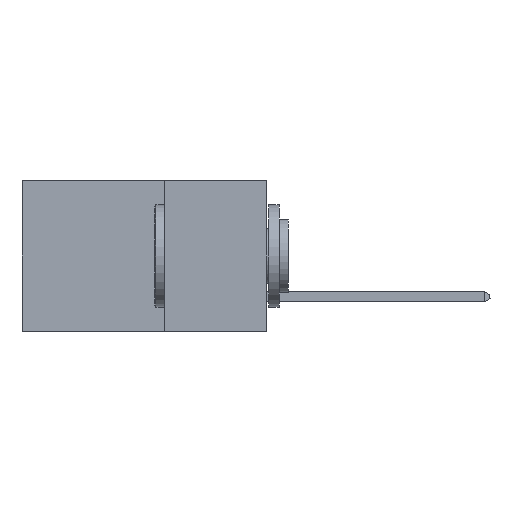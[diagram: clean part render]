
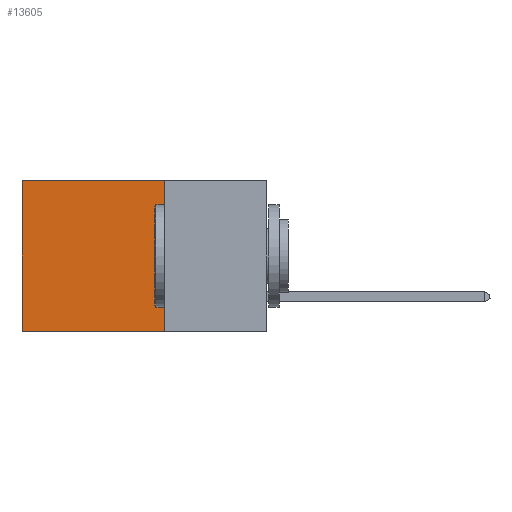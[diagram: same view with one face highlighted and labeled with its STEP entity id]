
A CAD part, left-side view. The second image highlights one B-rep face of the part: STEP entity #13605.
In plain terms, the highlighted planar face has unit normal (-1, 0, 0).
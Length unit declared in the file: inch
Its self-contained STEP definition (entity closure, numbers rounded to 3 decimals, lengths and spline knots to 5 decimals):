
#523 = FACE_OUTER_BOUND ( 'NONE', #15005, .T. ) ;
#1221 = DIRECTION ( 'NONE',  ( 1., 0., 0. ) ) ;
#2927 = LINE ( 'NONE', #26624, #24232 ) ;
#3961 = DIRECTION ( 'NONE',  ( 0., 1., 0. ) ) ;
#4845 = EDGE_CURVE ( 'NONE', #5559, #17962, #18027, .T. ) ;
#5559 = VERTEX_POINT ( 'NONE', #18708 ) ;
#5758 = AXIS2_PLACEMENT_3D ( 'NONE', #23909, #1221, #15977 ) ;
#5864 = CARTESIAN_POINT ( 'NONE',  ( 0.2875, 0.6, 0. ) ) ;
#5927 = ORIENTED_EDGE ( 'NONE', *, *, #7943, .F. ) ;
#7510 = VERTEX_POINT ( 'NONE', #18894 ) ;
#7943 = EDGE_CURVE ( 'NONE', #7510, #5559, #17322, .T. ) ;
#12088 = DIRECTION ( 'NONE',  ( 0., 0., -1. ) ) ;
#12649 = VECTOR ( 'NONE', #19004, 39.37008 ) ;
#13605 = ADVANCED_FACE ( 'NONE', ( #523 ), #15888, .F. ) ;
#15005 = EDGE_LOOP ( 'NONE', ( #26335, #26659, #5927, #25585 ) ) ;
#15888 = PLANE ( 'NONE',  #5758 ) ;
#15977 = DIRECTION ( 'NONE',  ( 0., 0., -1. ) ) ;
#16191 = LINE ( 'NONE', #26075, #16797 ) ;
#16797 = VECTOR ( 'NONE', #12088, 39.37008 ) ;
#16946 = EDGE_CURVE ( 'NONE', #23090, #17962, #16191, .T. ) ;
#16956 = CARTESIAN_POINT ( 'NONE',  ( 0.2875, 0.25, 0. ) ) ;
#17322 = LINE ( 'NONE', #16956, #12649 ) ;
#17962 = VERTEX_POINT ( 'NONE', #21613 ) ;
#18027 = LINE ( 'NONE', #18566, #23357 ) ;
#18305 = EDGE_CURVE ( 'NONE', #7510, #23090, #2927, .T. ) ;
#18566 = CARTESIAN_POINT ( 'NONE',  ( 0.2875, 0.25, -0.37 ) ) ;
#18704 = DIRECTION ( 'NONE',  ( 0., 1., 0. ) ) ;
#18708 = CARTESIAN_POINT ( 'NONE',  ( 0.2875, 0.25, -0.37 ) ) ;
#18894 = CARTESIAN_POINT ( 'NONE',  ( 0.2875, 0.25, 0. ) ) ;
#19004 = DIRECTION ( 'NONE',  ( 0., 0., -1. ) ) ;
#21613 = CARTESIAN_POINT ( 'NONE',  ( 0.2875, 0.6, -0.37 ) ) ;
#23090 = VERTEX_POINT ( 'NONE', #5864 ) ;
#23357 = VECTOR ( 'NONE', #3961, 39.37008 ) ;
#23909 = CARTESIAN_POINT ( 'NONE',  ( 0.2875, 0.25, 0. ) ) ;
#24232 = VECTOR ( 'NONE', #18704, 39.37008 ) ;
#25585 = ORIENTED_EDGE ( 'NONE', *, *, #18305, .T. ) ;
#26075 = CARTESIAN_POINT ( 'NONE',  ( 0.2875, 0.6, 0. ) ) ;
#26335 = ORIENTED_EDGE ( 'NONE', *, *, #16946, .T. ) ;
#26624 = CARTESIAN_POINT ( 'NONE',  ( 0.2875, 0.25, 0. ) ) ;
#26659 = ORIENTED_EDGE ( 'NONE', *, *, #4845, .F. ) ;
